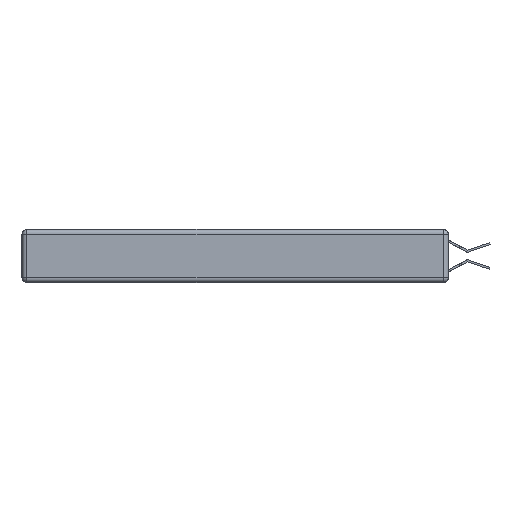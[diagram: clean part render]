
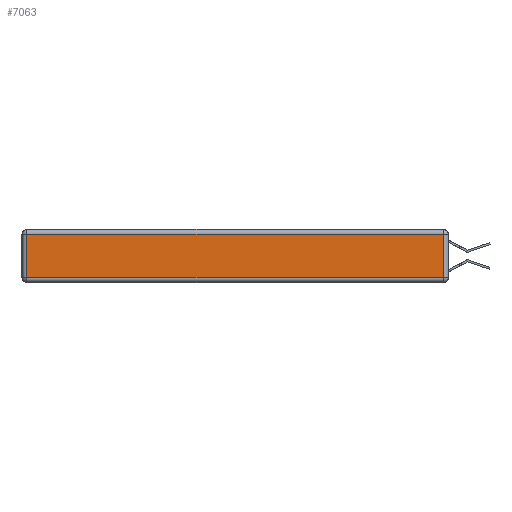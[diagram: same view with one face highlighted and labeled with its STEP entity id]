
A CAD part, left-side view. The second image highlights one B-rep face of the part: STEP entity #7063.
In plain terms, the highlighted planar face has unit normal (-1, 0, 0).
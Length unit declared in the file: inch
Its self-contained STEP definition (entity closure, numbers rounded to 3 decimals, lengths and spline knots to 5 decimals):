
#1175 = EDGE_CURVE ( 'NONE', #24275, #12410, #7776, .T. ) ;
#2205 = VECTOR ( 'NONE', #15692, 39.37008 ) ;
#2804 = CARTESIAN_POINT ( 'NONE',  ( 0., 0.03, -0.03 ) ) ;
#2855 = DIRECTION ( 'NONE',  ( 0., 0., 1. ) ) ;
#2907 = VECTOR ( 'NONE', #2855, 39.37008 ) ;
#3773 = VERTEX_POINT ( 'NONE', #16688 ) ;
#4578 = DIRECTION ( 'NONE',  ( 0., 0., 1. ) ) ;
#4711 = EDGE_LOOP ( 'NONE', ( #18083, #24326, #7753, #5524 ) ) ;
#5524 = ORIENTED_EDGE ( 'NONE', *, *, #9873, .T. ) ;
#7063 = ADVANCED_FACE ( 'NONE', ( #20442 ), #12733, .T. ) ;
#7753 = ORIENTED_EDGE ( 'NONE', *, *, #12472, .T. ) ;
#7776 = LINE ( 'NONE', #22275, #2907 ) ;
#8127 = EDGE_CURVE ( 'NONE', #3773, #24275, #17262, .T. ) ;
#9873 = EDGE_CURVE ( 'NONE', #24390, #3773, #10805, .T. ) ;
#10805 = LINE ( 'NONE', #19041, #26203 ) ;
#11037 = CARTESIAN_POINT ( 'NONE',  ( 0., 0.03, -0.313 ) ) ;
#11304 = VECTOR ( 'NONE', #24392, 39.37008 ) ;
#12410 = VERTEX_POINT ( 'NONE', #2804 ) ;
#12472 = EDGE_CURVE ( 'NONE', #12410, #24390, #23867, .T. ) ;
#12733 = PLANE ( 'NONE',  #19485 ) ;
#12998 = DIRECTION ( 'NONE',  ( 0., 0., -1. ) ) ;
#13653 = CARTESIAN_POINT ( 'NONE',  ( 0., 2.75, -0.03 ) ) ;
#15692 = DIRECTION ( 'NONE',  ( 0., 1., 0. ) ) ;
#16311 = CARTESIAN_POINT ( 'NONE',  ( 0., 0., -0.313 ) ) ;
#16688 = CARTESIAN_POINT ( 'NONE',  ( 0., 2.72, -0.313 ) ) ;
#16784 = DIRECTION ( 'NONE',  ( -1., 0., 0. ) ) ;
#17262 = LINE ( 'NONE', #16311, #11304 ) ;
#18083 = ORIENTED_EDGE ( 'NONE', *, *, #8127, .T. ) ;
#19041 = CARTESIAN_POINT ( 'NONE',  ( 0., 2.72, -0.343 ) ) ;
#19485 = AXIS2_PLACEMENT_3D ( 'NONE', #24801, #16784, #4578 ) ;
#20442 = FACE_OUTER_BOUND ( 'NONE', #4711, .T. ) ;
#22275 = CARTESIAN_POINT ( 'NONE',  ( 0., 0.03, -0.343 ) ) ;
#23867 = LINE ( 'NONE', #13653, #2205 ) ;
#24275 = VERTEX_POINT ( 'NONE', #11037 ) ;
#24326 = ORIENTED_EDGE ( 'NONE', *, *, #1175, .T. ) ;
#24390 = VERTEX_POINT ( 'NONE', #25428 ) ;
#24392 = DIRECTION ( 'NONE',  ( 0., -1., 0. ) ) ;
#24801 = CARTESIAN_POINT ( 'NONE',  ( 0., 0., -0.343 ) ) ;
#25428 = CARTESIAN_POINT ( 'NONE',  ( 0., 2.72, -0.03 ) ) ;
#26203 = VECTOR ( 'NONE', #12998, 39.37008 ) ;
